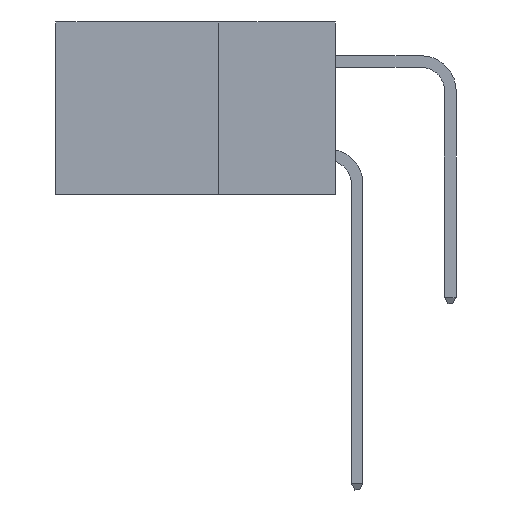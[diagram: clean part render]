
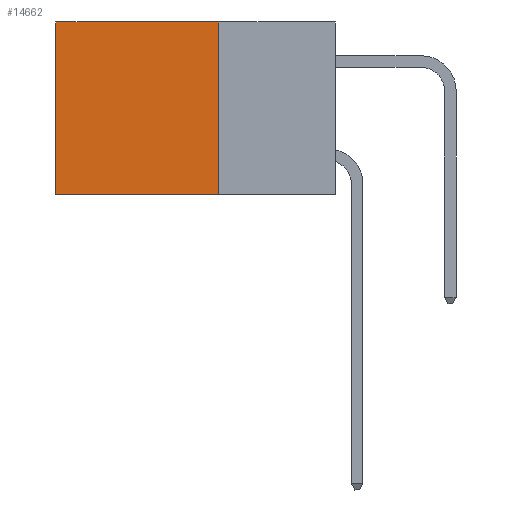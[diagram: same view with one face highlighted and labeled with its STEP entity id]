
A CAD part, left-side view. The second image highlights one B-rep face of the part: STEP entity #14662.
In plain terms, the highlighted planar face has unit normal (-1, 0, 0).
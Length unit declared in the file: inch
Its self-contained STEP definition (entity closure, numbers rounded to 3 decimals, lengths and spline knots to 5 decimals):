
#3194 = VERTEX_POINT ( 'NONE', #32397 ) ;
#6606 = CARTESIAN_POINT ( 'NONE',  ( 0.2875, 0.25, 0. ) ) ;
#6750 = DIRECTION ( 'NONE',  ( 0., 0., -1. ) ) ;
#7669 = CARTESIAN_POINT ( 'NONE',  ( 0.2875, 0.6, 0. ) ) ;
#7865 = ORIENTED_EDGE ( 'NONE', *, *, #7997, .T. ) ;
#7997 = EDGE_CURVE ( 'NONE', #3194, #19344, #41472, .T. ) ;
#8800 = VERTEX_POINT ( 'NONE', #37705 ) ;
#9313 = EDGE_CURVE ( 'NONE', #11316, #8800, #22132, .T. ) ;
#11099 = ORIENTED_EDGE ( 'NONE', *, *, #16576, .F. ) ;
#11316 = VERTEX_POINT ( 'NONE', #29769 ) ;
#12142 = VECTOR ( 'NONE', #27144, 39.37008 ) ;
#12842 = DIRECTION ( 'NONE',  ( 0., 0., -1. ) ) ;
#14662 = ADVANCED_FACE ( 'NONE', ( #38708 ), #25947, .F. ) ;
#16576 = EDGE_CURVE ( 'NONE', #3194, #11316, #26517, .T. ) ;
#17138 = VECTOR ( 'NONE', #40331, 39.37008 ) ;
#17938 = VECTOR ( 'NONE', #6750, 39.37008 ) ;
#19294 = VECTOR ( 'NONE', #37112, 39.37008 ) ;
#19344 = VERTEX_POINT ( 'NONE', #30372 ) ;
#21146 = CARTESIAN_POINT ( 'NONE',  ( 0.2875, 0.25, -0.37 ) ) ;
#22132 = LINE ( 'NONE', #21146, #17138 ) ;
#22965 = DIRECTION ( 'NONE',  ( 1., 0., 0. ) ) ;
#25947 = PLANE ( 'NONE',  #29264 ) ;
#26422 = ORIENTED_EDGE ( 'NONE', *, *, #26817, .T. ) ;
#26517 = LINE ( 'NONE', #32430, #17938 ) ;
#26817 = EDGE_CURVE ( 'NONE', #19344, #8800, #37902, .T. ) ;
#27144 = DIRECTION ( 'NONE',  ( 0., 0., -1. ) ) ;
#29264 = AXIS2_PLACEMENT_3D ( 'NONE', #6606, #22965, #12842 ) ;
#29769 = CARTESIAN_POINT ( 'NONE',  ( 0.2875, 0.25, -0.37 ) ) ;
#30372 = CARTESIAN_POINT ( 'NONE',  ( 0.2875, 0.6, 0. ) ) ;
#31032 = EDGE_LOOP ( 'NONE', ( #26422, #31338, #11099, #7865 ) ) ;
#31338 = ORIENTED_EDGE ( 'NONE', *, *, #9313, .F. ) ;
#32397 = CARTESIAN_POINT ( 'NONE',  ( 0.2875, 0.25, 0. ) ) ;
#32430 = CARTESIAN_POINT ( 'NONE',  ( 0.2875, 0.25, 0. ) ) ;
#36555 = CARTESIAN_POINT ( 'NONE',  ( 0.2875, 0.25, 0. ) ) ;
#37112 = DIRECTION ( 'NONE',  ( 0., 1., 0. ) ) ;
#37705 = CARTESIAN_POINT ( 'NONE',  ( 0.2875, 0.6, -0.37 ) ) ;
#37902 = LINE ( 'NONE', #7669, #12142 ) ;
#38708 = FACE_OUTER_BOUND ( 'NONE', #31032, .T. ) ;
#40331 = DIRECTION ( 'NONE',  ( 0., 1., 0. ) ) ;
#41472 = LINE ( 'NONE', #36555, #19294 ) ;
